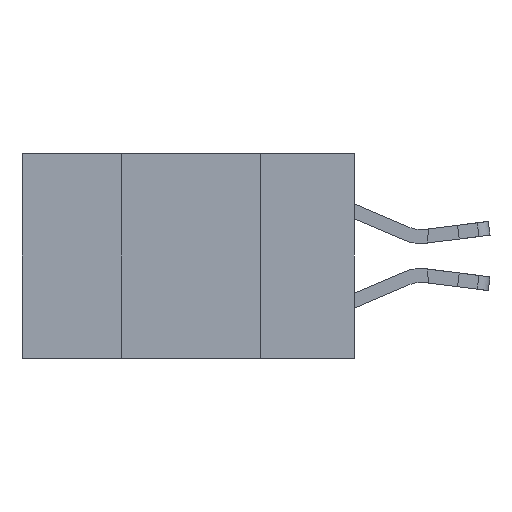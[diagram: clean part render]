
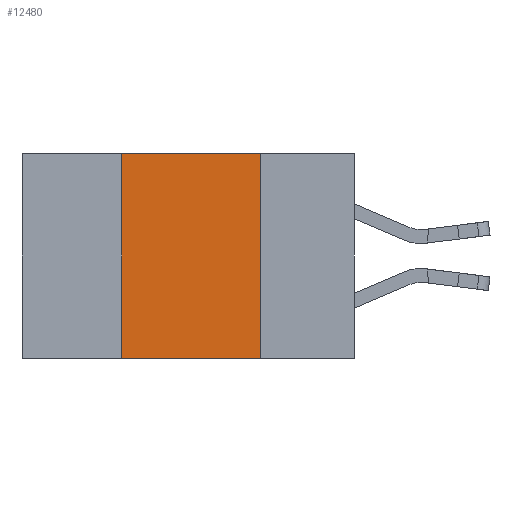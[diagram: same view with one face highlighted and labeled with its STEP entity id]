
A CAD part, left-side view. The second image highlights one B-rep face of the part: STEP entity #12480.
In plain terms, the highlighted planar face has unit normal (-1, 0, 0).
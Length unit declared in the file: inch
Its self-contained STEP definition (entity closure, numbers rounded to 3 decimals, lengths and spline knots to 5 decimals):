
#124 = AXIS2_PLACEMENT_3D ( 'NONE', #4653, #16937, #1038 ) ;
#1038 = DIRECTION ( 'NONE',  ( 0., 0., -1. ) ) ;
#1723 = DIRECTION ( 'NONE',  ( 0., 0., -1. ) ) ;
#1782 = EDGE_CURVE ( 'NONE', #12212, #19139, #4693, .T. ) ;
#2787 = FACE_OUTER_BOUND ( 'NONE', #16502, .T. ) ;
#3243 = EDGE_CURVE ( 'NONE', #19139, #20557, #4596, .T. ) ;
#4000 = VECTOR ( 'NONE', #11563, 39.37008 ) ;
#4196 = VECTOR ( 'NONE', #1723, 39.37008 ) ;
#4596 = LINE ( 'NONE', #18390, #4000 ) ;
#4653 = CARTESIAN_POINT ( 'NONE',  ( 0., 0.6, 0. ) ) ;
#4693 = LINE ( 'NONE', #17074, #16544 ) ;
#8378 = LINE ( 'NONE', #15201, #15051 ) ;
#8707 = LINE ( 'NONE', #11931, #4196 ) ;
#9292 = CARTESIAN_POINT ( 'NONE',  ( 0., 0.42, -0.37 ) ) ;
#9876 = PLANE ( 'NONE',  #124 ) ;
#10082 = CARTESIAN_POINT ( 'NONE',  ( 0., 0.17, 0. ) ) ;
#10218 = ORIENTED_EDGE ( 'NONE', *, *, #18933, .F. ) ;
#11563 = DIRECTION ( 'NONE',  ( 0., -1., 0. ) ) ;
#11713 = ORIENTED_EDGE ( 'NONE', *, *, #1782, .F. ) ;
#11931 = CARTESIAN_POINT ( 'NONE',  ( 0., 0.17, -0.37 ) ) ;
#12212 = VERTEX_POINT ( 'NONE', #9292 ) ;
#12480 = ADVANCED_FACE ( 'NONE', ( #2787 ), #9876, .F. ) ;
#13503 = ORIENTED_EDGE ( 'NONE', *, *, #15113, .T. ) ;
#15051 = VECTOR ( 'NONE', #19152, 39.37008 ) ;
#15113 = EDGE_CURVE ( 'NONE', #12212, #18663, #8378, .T. ) ;
#15201 = CARTESIAN_POINT ( 'NONE',  ( 0., 0.6, -0.37 ) ) ;
#16502 = EDGE_LOOP ( 'NONE', ( #10218, #22784, #11713, #13503 ) ) ;
#16544 = VECTOR ( 'NONE', #16861, 39.37008 ) ;
#16861 = DIRECTION ( 'NONE',  ( 0., 0., 1. ) ) ;
#16937 = DIRECTION ( 'NONE',  ( 1., 0., 0. ) ) ;
#17074 = CARTESIAN_POINT ( 'NONE',  ( 0., 0.42, -0.37 ) ) ;
#17216 = CARTESIAN_POINT ( 'NONE',  ( 0., 0.42, 0. ) ) ;
#18390 = CARTESIAN_POINT ( 'NONE',  ( 0., 0.6, 0. ) ) ;
#18663 = VERTEX_POINT ( 'NONE', #20518 ) ;
#18933 = EDGE_CURVE ( 'NONE', #20557, #18663, #8707, .T. ) ;
#19139 = VERTEX_POINT ( 'NONE', #17216 ) ;
#19152 = DIRECTION ( 'NONE',  ( 0., -1., 0. ) ) ;
#20518 = CARTESIAN_POINT ( 'NONE',  ( 0., 0.17, -0.37 ) ) ;
#20557 = VERTEX_POINT ( 'NONE', #10082 ) ;
#22784 = ORIENTED_EDGE ( 'NONE', *, *, #3243, .F. ) ;
